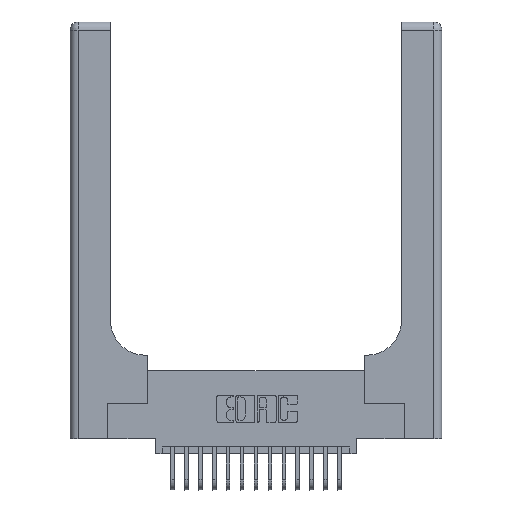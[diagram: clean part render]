
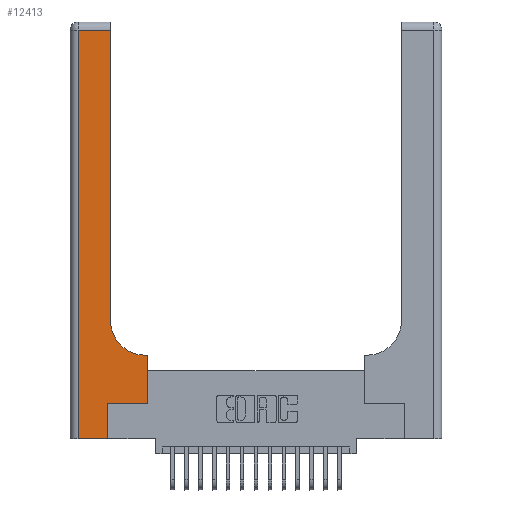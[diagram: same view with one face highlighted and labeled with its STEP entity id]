
A CAD part, top view. The second image highlights one B-rep face of the part: STEP entity #12413.
In plain terms, the highlighted planar face has unit normal (0, 0, 1).
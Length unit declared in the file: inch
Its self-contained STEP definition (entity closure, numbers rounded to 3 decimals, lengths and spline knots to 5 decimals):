
#303 = DIRECTION ( 'NONE',  ( 0., 0., -1. ) ) ;
#445 = CARTESIAN_POINT ( 'NONE',  ( 0.5415, 0.6, 0.37 ) ) ;
#488 = VERTEX_POINT ( 'NONE', #8466 ) ;
#760 = EDGE_LOOP ( 'NONE', ( #9552, #6782, #10267, #6919, #7003, #6162, #6392, #14151, #6541 ) ) ;
#1012 = DIRECTION ( 'NONE',  ( 0., 1., 0. ) ) ;
#1089 = VERTEX_POINT ( 'NONE', #445 ) ;
#1239 = DIRECTION ( 'NONE',  ( 0., 1., 0. ) ) ;
#1924 = PLANE ( 'NONE',  #6918 ) ;
#2122 = CIRCLE ( 'NONE', #4648, 0.25 ) ;
#2347 = VERTEX_POINT ( 'NONE', #5798 ) ;
#2643 = CARTESIAN_POINT ( 'NONE',  ( 0.2915, 2.94, 0.37 ) ) ;
#3036 = CARTESIAN_POINT ( 'NONE',  ( 0.269, 0., 0.37 ) ) ;
#3110 = CARTESIAN_POINT ( 'NONE',  ( 0.2915, 0.6, 0.37 ) ) ;
#3641 = VECTOR ( 'NONE', #5742, 39.37008 ) ;
#3718 = VECTOR ( 'NONE', #18858, 39.37008 ) ;
#4028 = VECTOR ( 'NONE', #11319, 39.37008 ) ;
#4203 = DIRECTION ( 'NONE',  ( 0., 0., -1. ) ) ;
#4648 = AXIS2_PLACEMENT_3D ( 'NONE', #14109, #4203, #15667 ) ;
#4770 = EDGE_CURVE ( 'NONE', #2347, #19453, #17081, .T. ) ;
#5100 = VERTEX_POINT ( 'NONE', #10572 ) ;
#5459 = VECTOR ( 'NONE', #10850, 39.37008 ) ;
#5742 = DIRECTION ( 'NONE',  ( 1., 0., 0. ) ) ;
#5798 = CARTESIAN_POINT ( 'NONE',  ( 0.5585, 0.25, 0.37 ) ) ;
#5865 = CARTESIAN_POINT ( 'NONE',  ( 0., 0., 0.37 ) ) ;
#5870 = CARTESIAN_POINT ( 'NONE',  ( 0.06, 2.94, 0.37 ) ) ;
#6162 = ORIENTED_EDGE ( 'NONE', *, *, #20273, .T. ) ;
#6380 = VECTOR ( 'NONE', #1012, 39.37008 ) ;
#6392 = ORIENTED_EDGE ( 'NONE', *, *, #4770, .T. ) ;
#6541 = ORIENTED_EDGE ( 'NONE', *, *, #18756, .T. ) ;
#6782 = ORIENTED_EDGE ( 'NONE', *, *, #8874, .T. ) ;
#6918 = AXIS2_PLACEMENT_3D ( 'NONE', #8580, #303, #11925 ) ;
#6919 = ORIENTED_EDGE ( 'NONE', *, *, #17734, .T. ) ;
#6982 = VERTEX_POINT ( 'NONE', #5870 ) ;
#7003 = ORIENTED_EDGE ( 'NONE', *, *, #14980, .T. ) ;
#8089 = DIRECTION ( 'NONE',  ( -1., 0., 0. ) ) ;
#8466 = CARTESIAN_POINT ( 'NONE',  ( 0.2915, 0.85, 0.37 ) ) ;
#8577 = EDGE_CURVE ( 'NONE', #6982, #14897, #19191, .T. ) ;
#8580 = CARTESIAN_POINT ( 'NONE',  ( 0., 3., 0.37 ) ) ;
#8874 = EDGE_CURVE ( 'NONE', #16602, #6982, #17950, .T. ) ;
#9552 = ORIENTED_EDGE ( 'NONE', *, *, #9708, .T. ) ;
#9708 = EDGE_CURVE ( 'NONE', #488, #16602, #20362, .T. ) ;
#10267 = ORIENTED_EDGE ( 'NONE', *, *, #8577, .T. ) ;
#10572 = CARTESIAN_POINT ( 'NONE',  ( 0.269, 0.25, 0.37 ) ) ;
#10779 = LINE ( 'NONE', #17370, #6380 ) ;
#10850 = DIRECTION ( 'NONE',  ( -1., 0., 0. ) ) ;
#11319 = DIRECTION ( 'NONE',  ( 0., 1., 0. ) ) ;
#11925 = DIRECTION ( 'NONE',  ( -1., 0., 0. ) ) ;
#12413 = ADVANCED_FACE ( 'NONE', ( #14200 ), #1924, .F. ) ;
#12418 = CARTESIAN_POINT ( 'NONE',  ( 0.06, 0., 0.37 ) ) ;
#12956 = CARTESIAN_POINT ( 'NONE',  ( 0.5585, 0.25, 0.37 ) ) ;
#13162 = CARTESIAN_POINT ( 'NONE',  ( 0.06, 3., 0.37 ) ) ;
#13291 = CARTESIAN_POINT ( 'NONE',  ( 0.5585, 0.6, 0.37 ) ) ;
#13493 = LINE ( 'NONE', #15536, #3641 ) ;
#13845 = LINE ( 'NONE', #3110, #17561 ) ;
#13855 = VERTEX_POINT ( 'NONE', #3036 ) ;
#14109 = CARTESIAN_POINT ( 'NONE',  ( 0.5415, 0.85, 0.37 ) ) ;
#14151 = ORIENTED_EDGE ( 'NONE', *, *, #15726, .T. ) ;
#14200 = FACE_OUTER_BOUND ( 'NONE', #760, .T. ) ;
#14897 = VERTEX_POINT ( 'NONE', #12418 ) ;
#14969 = VECTOR ( 'NONE', #17970, 39.37008 ) ;
#14980 = EDGE_CURVE ( 'NONE', #13855, #5100, #10779, .T. ) ;
#15536 = CARTESIAN_POINT ( 'NONE',  ( 0.269, 0.25, 0.37 ) ) ;
#15661 = VECTOR ( 'NONE', #1239, 39.37008 ) ;
#15667 = DIRECTION ( 'NONE',  ( 1., 0., 0. ) ) ;
#15726 = EDGE_CURVE ( 'NONE', #19453, #1089, #13845, .T. ) ;
#16602 = VERTEX_POINT ( 'NONE', #2643 ) ;
#16772 = LINE ( 'NONE', #5865, #3718 ) ;
#17081 = LINE ( 'NONE', #12956, #4028 ) ;
#17370 = CARTESIAN_POINT ( 'NONE',  ( 0.269, 0., 0.37 ) ) ;
#17561 = VECTOR ( 'NONE', #8089, 39.37008 ) ;
#17734 = EDGE_CURVE ( 'NONE', #14897, #13855, #16772, .T. ) ;
#17950 = LINE ( 'NONE', #20408, #5459 ) ;
#17970 = DIRECTION ( 'NONE',  ( 0., -1., 0. ) ) ;
#18756 = EDGE_CURVE ( 'NONE', #1089, #488, #2122, .T. ) ;
#18858 = DIRECTION ( 'NONE',  ( 1., 0., 0. ) ) ;
#19191 = LINE ( 'NONE', #13162, #14969 ) ;
#19453 = VERTEX_POINT ( 'NONE', #13291 ) ;
#20273 = EDGE_CURVE ( 'NONE', #5100, #2347, #13493, .T. ) ;
#20362 = LINE ( 'NONE', #20727, #15661 ) ;
#20408 = CARTESIAN_POINT ( 'NONE',  ( 0., 2.94, 0.37 ) ) ;
#20727 = CARTESIAN_POINT ( 'NONE',  ( 0.2915, 3., 0.37 ) ) ;
